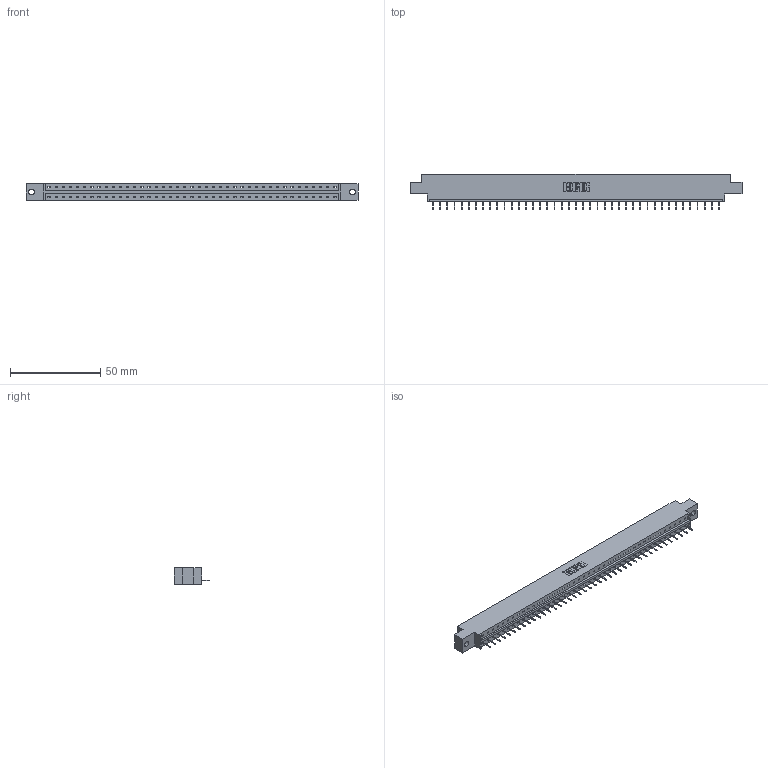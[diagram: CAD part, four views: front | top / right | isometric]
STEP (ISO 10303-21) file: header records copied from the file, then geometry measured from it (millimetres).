
FILE_DESCRIPTION (( 'STEP AP203' ), '1' );
FILE_NAME ('833-041-524-602.STEP', '2020-06-03T19:02:27', ( '' ), ( '' ), 'SwSTEP 2.0', 'SolidWorks 2020', '' );
FILE_SCHEMA (( 'CONFIG_CONTROL_DESIGN' ));
Length unit declared in the file: inch
Products named in the file (3): 833-041-524-602; 345-292-001_345-293-124; 833 Part_Offset - .128 Dia
Assembly tree (42 placements, depth 2):
  833-041-524-602
    833 Part_Offset - .128 Dia
    345-292-001_345-293-124  x41
Bounding box: 184 x 19.69 x 9.4 mm (x, y, z)
Volume: 18080.3 mm3; surface area: 18925.2 mm2
Topology: 42 solids, 42 shells, 2660 faces, 7703 edges, 4970 vertices
Faces by surface type: plane 2042, cylinder 618
Entity records: 25403 total; most frequent: CARTESIAN_POINT 4389, ORIENTED_EDGE 4366, DIRECTION 3705, EDGE_CURVE 2183, VECTOR 2059, LINE 2059, VERTEX_POINT 1450, AXIS2_PLACEMENT_3D 823
